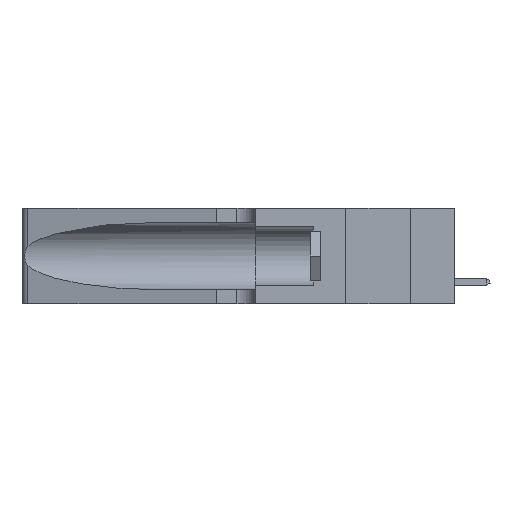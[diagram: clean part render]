
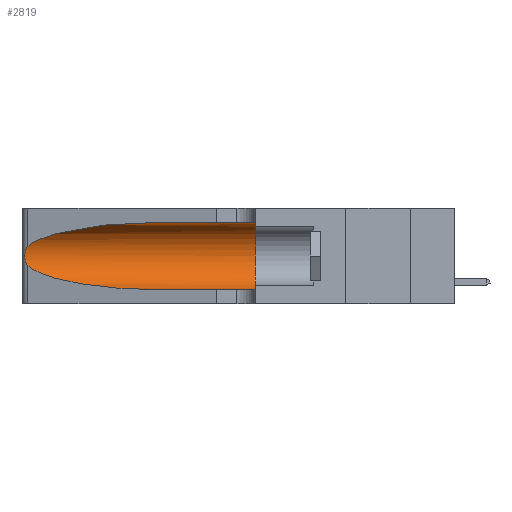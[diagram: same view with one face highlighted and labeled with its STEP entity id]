
A CAD part, left-side view. The second image highlights one B-rep face of the part: STEP entity #2819.
In plain terms, the highlighted cylindrical face has radius 3.308 mm (diameter 6.617 mm), a partial arc.
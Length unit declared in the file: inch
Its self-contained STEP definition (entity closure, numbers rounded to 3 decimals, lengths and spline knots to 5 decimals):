
#85 = CARTESIAN_POINT ( 'NONE',  ( 0.26018, 1.23835, 0.19895 ) ) ;
#148 = CARTESIAN_POINT ( 'NONE',  ( 0.25789, 1.23486, 0.15765 ) ) ;
#511 = VECTOR ( 'NONE', #21975, 39.37008 ) ;
#1257 = ORIENTED_EDGE ( 'NONE', *, *, #14133, .T. ) ;
#1469 = CARTESIAN_POINT ( 'NONE',  ( 0.1305, 0.72297, 0.31525 ) ) ;
#1490 = DIRECTION ( 'NONE',  ( 0., 0., 1. ) ) ;
#1709 = VERTEX_POINT ( 'NONE', #3902 ) ;
#2056 = CARTESIAN_POINT ( 'NONE',  ( 0.26075, 1.23896, 0.178 ) ) ;
#2819 = ADVANCED_FACE ( 'NONE', ( #4237 ), #19475, .F. ) ;
#2907 = CARTESIAN_POINT ( 'NONE',  ( 0.1305, 0.35, 0.185 ) ) ;
#3279 = CARTESIAN_POINT ( 'NONE',  ( 0.18966, 0.96281, 0.05475 ) ) ;
#3300 = LINE ( 'NONE', #8343, #511 ) ;
#3902 = CARTESIAN_POINT ( 'NONE',  ( 0.25487, 1.22718, 0.14631 ) ) ;
#4237 = FACE_OUTER_BOUND ( 'NONE', #12587, .T. ) ;
#4462 = ORIENTED_EDGE ( 'NONE', *, *, #15575, .F. ) ;
#4879 = VECTOR ( 'NONE', #16990, 39.37008 ) ;
#5061 = VERTEX_POINT ( 'NONE', #18354 ) ;
#5129 = CARTESIAN_POINT ( 'NONE',  ( 0.1305, 1.61858, 0.05475 ) ) ;
#5163 = ORIENTED_EDGE ( 'NONE', *, *, #16146, .T. ) ;
#5535 = EDGE_CURVE ( 'NONE', #14967, #5061, #20551, .T. ) ;
#6110 = CARTESIAN_POINT ( 'NONE',  ( 0.18966, 0.96281, 0.31525 ) ) ;
#6120 = CARTESIAN_POINT ( 'NONE',  ( 0.25639, 1.23184, 0.21858 ) ) ;
#6753 = DIRECTION ( 'NONE',  ( 0., 0., -1. ) ) ;
#7462 = CARTESIAN_POINT ( 'NONE',  ( 0.1305, 0.72297, 0.05475 ) ) ;
#7699 = VERTEX_POINT ( 'NONE', #13098 ) ;
#7856 = CARTESIAN_POINT ( 'NONE',  ( 0.25487, 1.22718, 0.22369 ) ) ;
#8006 = CARTESIAN_POINT ( 'NONE',  ( 0.25787, 1.23484, 0.2124 ) ) ;
#8343 = CARTESIAN_POINT ( 'NONE',  ( 0.1305, 1.61858, 0.31525 ) ) ;
#9074 = ORIENTED_EDGE ( 'NONE', *, *, #5535, .F. ) ;
#9454 = EDGE_CURVE ( 'NONE', #17263, #5061, #22272, .T. ) ;
#9812 = CARTESIAN_POINT ( 'NONE',  ( 0.26075, 1.23896, 0.19203 ) ) ;
#10110 = CARTESIAN_POINT ( 'NONE',  ( 0.25555, 1.22993, 0.14849 ) ) ;
#10451 = AXIS2_PLACEMENT_3D ( 'NONE', #16134, #20038, #6753 ) ;
#12587 = EDGE_LOOP ( 'NONE', ( #5163, #16413, #1257, #22568, #9074, #4462 ) ) ;
#13098 = CARTESIAN_POINT ( 'NONE',  ( 0.25487, 1.22718, 0.22369 ) ) ;
#13739 = CARTESIAN_POINT ( 'NONE',  ( 0.25854, 1.2359, 0.20912 ) ) ;
#13807 = CARTESIAN_POINT ( 'NONE',  ( 0.1305, 0.72297, 0.31525 ) ) ;
#13815 = CARTESIAN_POINT ( 'NONE',  ( 0.25487, 1.22718, 0.14631 ) ) ;
#14052 = CARTESIAN_POINT ( 'NONE',  ( 0.25639, 1.23186, 0.15144 ) ) ;
#14133 = EDGE_CURVE ( 'NONE', #1709, #17263, #16546, .T. ) ;
#14203 = CARTESIAN_POINT ( 'NONE',  ( 0.25487, 1.22718, 0.22369 ) ) ;
#14967 = VERTEX_POINT ( 'NONE', #21667 ) ;
#14982 = CARTESIAN_POINT ( 'NONE',  ( 0.2373, 1.15595, 0.08982 ) ) ;
#15487 =( BOUNDED_CURVE ( )  B_SPLINE_CURVE ( 3, ( #13807, #6110, #23759, #14203 ),
 .UNSPECIFIED., .F., .F. ) 
 B_SPLINE_CURVE_WITH_KNOTS ( ( 4, 4 ),
 ( 1.5708, 2.84003 ),
 .UNSPECIFIED. ) 
 CURVE ( )  GEOMETRIC_REPRESENTATION_ITEM ( )  RATIONAL_B_SPLINE_CURVE ( ( 1., 0.87, 0.87, 1. ) ) 
 REPRESENTATION_ITEM ( '' )  );
#15575 = EDGE_CURVE ( 'NONE', #19645, #14967, #3300, .T. ) ;
#15852 = CARTESIAN_POINT ( 'NONE',  ( 0.25856, 1.23593, 0.16098 ) ) ;
#16134 = CARTESIAN_POINT ( 'NONE',  ( 0.1305, 1.61858, 0.185 ) ) ;
#16146 = EDGE_CURVE ( 'NONE', #19645, #7699, #15487, .T. ) ;
#16413 = ORIENTED_EDGE ( 'NONE', *, *, #24170, .T. ) ;
#16546 =( BOUNDED_CURVE ( )  B_SPLINE_CURVE ( 3, ( #22719, #14982, #3279, #7462 ),
 .UNSPECIFIED., .F., .T. ) 
 B_SPLINE_CURVE_WITH_KNOTS ( ( 4, 4 ),
 ( 3.44316, 4.71239 ),
 .UNSPECIFIED. ) 
 CURVE ( )  GEOMETRIC_REPRESENTATION_ITEM ( )  RATIONAL_B_SPLINE_CURVE ( ( 1., 0.87, 0.87, 1. ) ) 
 REPRESENTATION_ITEM ( '' )  );
#16990 = DIRECTION ( 'NONE',  ( 0., -1., 0. ) ) ;
#17263 = VERTEX_POINT ( 'NONE', #18053 ) ;
#17780 = CARTESIAN_POINT ( 'NONE',  ( 0.26017, 1.23833, 0.17102 ) ) ;
#18053 = CARTESIAN_POINT ( 'NONE',  ( 0.1305, 0.72297, 0.05475 ) ) ;
#18354 = CARTESIAN_POINT ( 'NONE',  ( 0.1305, 0.35, 0.05475 ) ) ;
#18492 = DIRECTION ( 'NONE',  ( 0., 1., 0. ) ) ;
#19475 = CYLINDRICAL_SURFACE ( 'NONE', #10451, 0.13025 ) ;
#19645 = VERTEX_POINT ( 'NONE', #1469 ) ;
#19827 = CARTESIAN_POINT ( 'NONE',  ( 0.25555, 1.22994, 0.2215 ) ) ;
#20038 = DIRECTION ( 'NONE',  ( 0., -1., 0. ) ) ;
#20551 = CIRCLE ( 'NONE', #22632, 0.13025 ) ;
#21667 = CARTESIAN_POINT ( 'NONE',  ( 0.1305, 0.35, 0.31525 ) ) ;
#21975 = DIRECTION ( 'NONE',  ( 0., -1., 0. ) ) ;
#22272 = LINE ( 'NONE', #5129, #4879 ) ;
#22568 = ORIENTED_EDGE ( 'NONE', *, *, #9454, .T. ) ;
#22632 = AXIS2_PLACEMENT_3D ( 'NONE', #2907, #18492, #1490 ) ;
#22719 = CARTESIAN_POINT ( 'NONE',  ( 0.25487, 1.22718, 0.14631 ) ) ;
#23759 = CARTESIAN_POINT ( 'NONE',  ( 0.2373, 1.15595, 0.28018 ) ) ;
#24053 = B_SPLINE_CURVE_WITH_KNOTS ( 'NONE', 3,
 ( #7856, #19827, #6120, #8006, #13739, #85, #9812, #2056, #17780, #15852, #148, #14052, #10110, #13815 ),
 .UNSPECIFIED., .F., .F.,
 ( 4, 2, 2, 2, 2, 2, 4 ),
 ( 0., 0.00027, 0.00053, 0.00107, 0.0016, 0.00187, 0.00214 ),
 .UNSPECIFIED. ) ;
#24170 = EDGE_CURVE ( 'NONE', #7699, #1709, #24053, .T. ) ;
